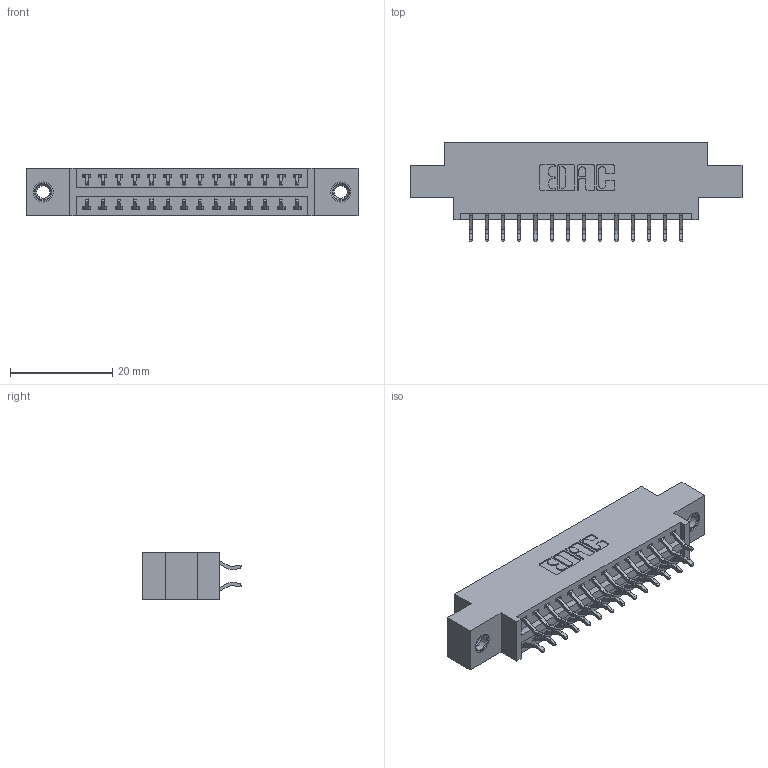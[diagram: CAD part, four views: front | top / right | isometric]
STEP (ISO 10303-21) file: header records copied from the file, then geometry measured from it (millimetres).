
FILE_DESCRIPTION (( 'STEP AP203' ), '1' );
FILE_NAME ('396-028-556-807.STEP', '2018-09-05T04:03:35', ( '' ), ( '' ), 'SwSTEP 2.0', 'SolidWorks 2016', '' );
FILE_SCHEMA (( 'CONFIG_CONTROL_DESIGN' ));
Length unit declared in the file: inch
Products named in the file (4): 346 Part_0.170 Offset - 0.156 Dia-TI; 345-292-001_556 Tail; 345-250-001_345-250-005-103; 396-028-556-807
Assembly tree (31 placements, depth 2):
  396-028-556-807
    346 Part_0.170 Offset - 0.156 Dia-TI
    345-292-001_556 Tail  x28
    345-250-001_345-250-005-103  x2
Bounding box: 65.02 x 19.57 x 9.4 mm (x, y, z)
Volume: 5953.9 mm3; surface area: 7931.4 mm2
Topology: 31 solids, 31 shells, 1810 faces, 5321 edges, 3502 vertices
Faces by surface type: plane 1204, cylinder 590, cone 12, torus 4
Entity records: 14444 total; most frequent: CARTESIAN_POINT 2419, ORIENTED_EDGE 2334, DIRECTION 2197, EDGE_CURVE 1167, VECTOR 951, LINE 951, VERTEX_POINT 772, AXIS2_PLACEMENT_3D 623
